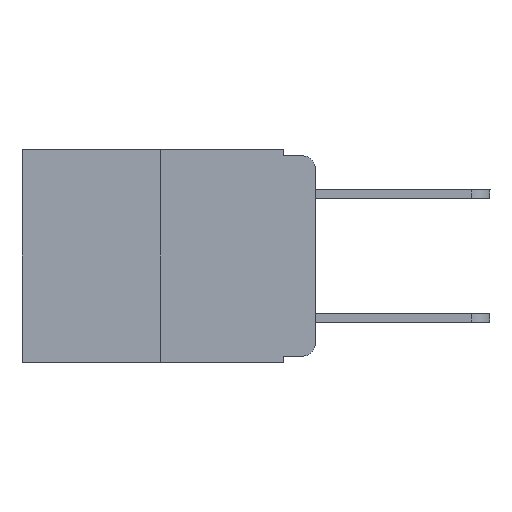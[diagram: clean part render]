
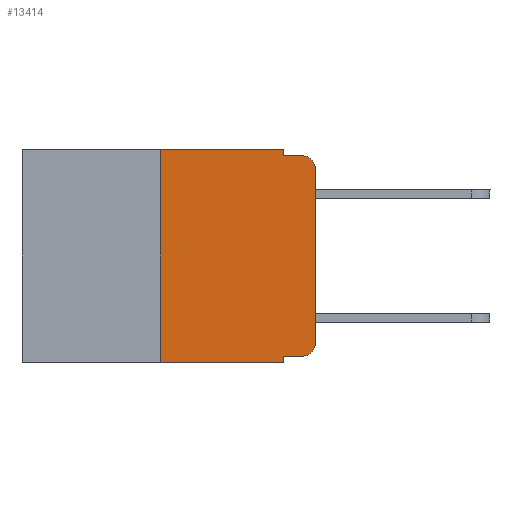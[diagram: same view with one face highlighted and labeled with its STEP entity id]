
A CAD part, left-side view. The second image highlights one B-rep face of the part: STEP entity #13414.
In plain terms, the highlighted planar face has unit normal (-1, 0, 0).
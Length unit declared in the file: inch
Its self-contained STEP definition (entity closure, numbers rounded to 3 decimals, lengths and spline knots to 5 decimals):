
#28 = DIRECTION ( 'NONE',  ( 0., -1., 0. ) ) ;
#113 = VECTOR ( 'NONE', #3943, 39.37008 ) ;
#271 = EDGE_CURVE ( 'NONE', #7825, #14316, #4235, .T. ) ;
#296 = EDGE_CURVE ( 'NONE', #1956, #3188, #5534, .T. ) ;
#317 = ORIENTED_EDGE ( 'NONE', *, *, #9508, .T. ) ;
#379 = VERTEX_POINT ( 'NONE', #7094 ) ;
#430 = LINE ( 'NONE', #10690, #527 ) ;
#527 = VECTOR ( 'NONE', #5223, 39.37008 ) ;
#608 = AXIS2_PLACEMENT_3D ( 'NONE', #4891, #9445, #13993 ) ;
#681 = CARTESIAN_POINT ( 'NONE',  ( 0., 0.051, -0.01 ) ) ;
#722 = DIRECTION ( 'NONE',  ( 0., -1., 0. ) ) ;
#794 = VECTOR ( 'NONE', #13948, 39.37008 ) ;
#1379 = EDGE_CURVE ( 'NONE', #10770, #7825, #14047, .T. ) ;
#1457 = CARTESIAN_POINT ( 'NONE',  ( 0., 0.051, 0. ) ) ;
#1654 = CARTESIAN_POINT ( 'NONE',  ( 0., 0.25, 0. ) ) ;
#1956 = VERTEX_POINT ( 'NONE', #12009 ) ;
#2827 = EDGE_CURVE ( 'NONE', #8071, #1956, #5105, .T. ) ;
#3049 = CARTESIAN_POINT ( 'NONE',  ( 0., 0.02, -0.03 ) ) ;
#3188 = VERTEX_POINT ( 'NONE', #12912 ) ;
#3722 = CARTESIAN_POINT ( 'NONE',  ( 0., 0., 0. ) ) ;
#3788 = EDGE_CURVE ( 'NONE', #8071, #8364, #6612, .T. ) ;
#3865 = CARTESIAN_POINT ( 'NONE',  ( 0., 0.051, -0.01 ) ) ;
#3943 = DIRECTION ( 'NONE',  ( 0., 0., 1. ) ) ;
#4164 = CARTESIAN_POINT ( 'NONE',  ( 0., 0., -0.313 ) ) ;
#4235 = CIRCLE ( 'NONE', #10695, 0.02 ) ;
#4519 = CARTESIAN_POINT ( 'NONE',  ( 0., 0.473, -0.343 ) ) ;
#4586 = ORIENTED_EDGE ( 'NONE', *, *, #3788, .T. ) ;
#4589 = DIRECTION ( 'NONE',  ( 0., 0., -1. ) ) ;
#4821 = ORIENTED_EDGE ( 'NONE', *, *, #1379, .T. ) ;
#4891 = CARTESIAN_POINT ( 'NONE',  ( 0., 0.02, -0.313 ) ) ;
#4953 = ORIENTED_EDGE ( 'NONE', *, *, #14022, .F. ) ;
#5105 = LINE ( 'NONE', #1654, #6030 ) ;
#5132 = AXIS2_PLACEMENT_3D ( 'NONE', #6598, #7848, #4589 ) ;
#5223 = DIRECTION ( 'NONE',  ( 0., -1., 0. ) ) ;
#5534 = LINE ( 'NONE', #10992, #11641 ) ;
#5621 = VECTOR ( 'NONE', #10986, 39.37008 ) ;
#5875 = ORIENTED_EDGE ( 'NONE', *, *, #11196, .F. ) ;
#6030 = VECTOR ( 'NONE', #8387, 39.37008 ) ;
#6242 = CARTESIAN_POINT ( 'NONE',  ( 0., 0.02, -0.01 ) ) ;
#6566 = VECTOR ( 'NONE', #28, 39.37008 ) ;
#6598 = CARTESIAN_POINT ( 'NONE',  ( 0., 0.473, 0. ) ) ;
#6612 = LINE ( 'NONE', #4519, #6566 ) ;
#6658 = VERTEX_POINT ( 'NONE', #12434 ) ;
#7094 = CARTESIAN_POINT ( 'NONE',  ( 0., 0.051, -0.333 ) ) ;
#7778 = PLANE ( 'NONE',  #5132 ) ;
#7825 = VERTEX_POINT ( 'NONE', #13042 ) ;
#7848 = DIRECTION ( 'NONE',  ( 1., 0., 0. ) ) ;
#7928 = FACE_OUTER_BOUND ( 'NONE', #12571, .T. ) ;
#8071 = VERTEX_POINT ( 'NONE', #10491 ) ;
#8364 = VERTEX_POINT ( 'NONE', #11013 ) ;
#8387 = DIRECTION ( 'NONE',  ( 0., 0., 1. ) ) ;
#8871 = ORIENTED_EDGE ( 'NONE', *, *, #271, .T. ) ;
#9031 = DIRECTION ( 'NONE',  ( 0., 0., -1. ) ) ;
#9445 = DIRECTION ( 'NONE',  ( -1., 0., 0. ) ) ;
#9468 = CIRCLE ( 'NONE', #608, 0.02 ) ;
#9508 = EDGE_CURVE ( 'NONE', #379, #6658, #430, .T. ) ;
#9862 = EDGE_CURVE ( 'NONE', #3188, #14416, #10354, .T. ) ;
#10344 = ORIENTED_EDGE ( 'NONE', *, *, #14772, .T. ) ;
#10354 = LINE ( 'NONE', #1457, #13663 ) ;
#10491 = CARTESIAN_POINT ( 'NONE',  ( 0., 0.25, -0.343 ) ) ;
#10591 = CARTESIAN_POINT ( 'NONE',  ( 0., 0.051, 0. ) ) ;
#10690 = CARTESIAN_POINT ( 'NONE',  ( 0., 0.051, -0.333 ) ) ;
#10695 = AXIS2_PLACEMENT_3D ( 'NONE', #3049, #14488, #9031 ) ;
#10770 = VERTEX_POINT ( 'NONE', #4164 ) ;
#10796 = ORIENTED_EDGE ( 'NONE', *, *, #2827, .F. ) ;
#10986 = DIRECTION ( 'NONE',  ( 0., -1., 0. ) ) ;
#10992 = CARTESIAN_POINT ( 'NONE',  ( 0., 0.473, 0. ) ) ;
#11013 = CARTESIAN_POINT ( 'NONE',  ( 0., 0.051, -0.343 ) ) ;
#11196 = EDGE_CURVE ( 'NONE', #379, #8364, #12834, .T. ) ;
#11381 = ORIENTED_EDGE ( 'NONE', *, *, #9862, .F. ) ;
#11410 = DIRECTION ( 'NONE',  ( 0., 0., -1. ) ) ;
#11641 = VECTOR ( 'NONE', #722, 39.37008 ) ;
#11743 = ORIENTED_EDGE ( 'NONE', *, *, #296, .F. ) ;
#12009 = CARTESIAN_POINT ( 'NONE',  ( 0., 0.25, 0. ) ) ;
#12434 = CARTESIAN_POINT ( 'NONE',  ( 0., 0.02, -0.333 ) ) ;
#12571 = EDGE_LOOP ( 'NONE', ( #4821, #8871, #4953, #11381, #11743, #10796, #4586, #5875, #317, #10344 ) ) ;
#12834 = LINE ( 'NONE', #10591, #794 ) ;
#12912 = CARTESIAN_POINT ( 'NONE',  ( 0., 0.051, 0. ) ) ;
#12998 = LINE ( 'NONE', #3865, #5621 ) ;
#13042 = CARTESIAN_POINT ( 'NONE',  ( 0., 0., -0.03 ) ) ;
#13414 = ADVANCED_FACE ( 'NONE', ( #7928 ), #7778, .F. ) ;
#13663 = VECTOR ( 'NONE', #11410, 39.37008 ) ;
#13948 = DIRECTION ( 'NONE',  ( 0., 0., -1. ) ) ;
#13993 = DIRECTION ( 'NONE',  ( 0., 0., -1. ) ) ;
#14022 = EDGE_CURVE ( 'NONE', #14416, #14316, #12998, .T. ) ;
#14047 = LINE ( 'NONE', #3722, #113 ) ;
#14316 = VERTEX_POINT ( 'NONE', #6242 ) ;
#14416 = VERTEX_POINT ( 'NONE', #681 ) ;
#14488 = DIRECTION ( 'NONE',  ( -1., 0., 0. ) ) ;
#14772 = EDGE_CURVE ( 'NONE', #6658, #10770, #9468, .T. ) ;
